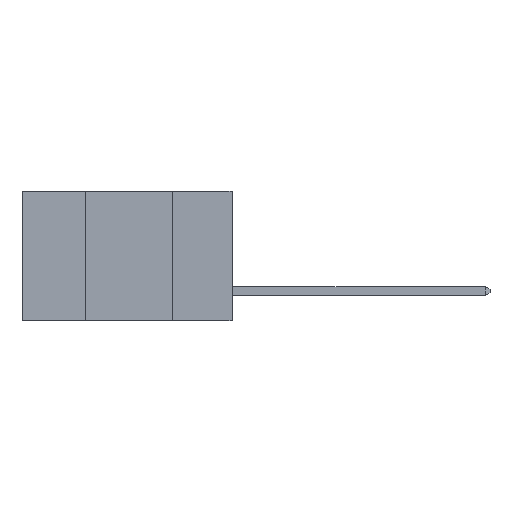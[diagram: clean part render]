
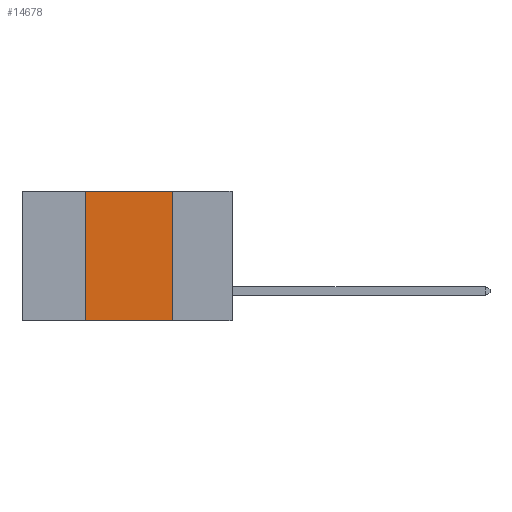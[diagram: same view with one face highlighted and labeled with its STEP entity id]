
A CAD part, left-side view. The second image highlights one B-rep face of the part: STEP entity #14678.
In plain terms, the highlighted planar face has unit normal (-1, 0, 0).
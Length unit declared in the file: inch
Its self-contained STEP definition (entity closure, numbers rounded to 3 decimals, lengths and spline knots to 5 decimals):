
#49 = DIRECTION ( 'NONE',  ( 0., -1., 0. ) ) ;
#316 = EDGE_CURVE ( 'NONE', #16548, #1294, #3854, .T. ) ;
#1294 = VERTEX_POINT ( 'NONE', #8686 ) ;
#1360 = ORIENTED_EDGE ( 'NONE', *, *, #15872, .F. ) ;
#1593 = LINE ( 'NONE', #1700, #14858 ) ;
#1700 = CARTESIAN_POINT ( 'NONE',  ( 0., 0.6, 0. ) ) ;
#1778 = VECTOR ( 'NONE', #7247, 39.37008 ) ;
#2514 = EDGE_LOOP ( 'NONE', ( #7907, #14664, #1360, #8323 ) ) ;
#3854 = LINE ( 'NONE', #7287, #13707 ) ;
#4302 = DIRECTION ( 'NONE',  ( 0., -1., 0. ) ) ;
#4315 = AXIS2_PLACEMENT_3D ( 'NONE', #5778, #14740, #7105 ) ;
#4480 = PLANE ( 'NONE',  #4315 ) ;
#5778 = CARTESIAN_POINT ( 'NONE',  ( 0., 0.6, 0. ) ) ;
#7105 = DIRECTION ( 'NONE',  ( 0., 0., -1. ) ) ;
#7247 = DIRECTION ( 'NONE',  ( 0., 0., 1. ) ) ;
#7287 = CARTESIAN_POINT ( 'NONE',  ( 0., 0.6, -0.37 ) ) ;
#7333 = CARTESIAN_POINT ( 'NONE',  ( 0., 0.42, 0. ) ) ;
#7784 = EDGE_CURVE ( 'NONE', #11010, #14756, #1593, .T. ) ;
#7906 = EDGE_CURVE ( 'NONE', #14756, #1294, #16605, .T. ) ;
#7907 = ORIENTED_EDGE ( 'NONE', *, *, #7906, .F. ) ;
#8169 = CARTESIAN_POINT ( 'NONE',  ( 0., 0.17, 0. ) ) ;
#8323 = ORIENTED_EDGE ( 'NONE', *, *, #316, .T. ) ;
#8686 = CARTESIAN_POINT ( 'NONE',  ( 0., 0.17, -0.37 ) ) ;
#11010 = VERTEX_POINT ( 'NONE', #7333 ) ;
#11124 = CARTESIAN_POINT ( 'NONE',  ( 0., 0.42, -0.37 ) ) ;
#11743 = FACE_OUTER_BOUND ( 'NONE', #2514, .T. ) ;
#12021 = DIRECTION ( 'NONE',  ( 0., 0., -1. ) ) ;
#12340 = CARTESIAN_POINT ( 'NONE',  ( 0., 0.42, 0. ) ) ;
#12374 = CARTESIAN_POINT ( 'NONE',  ( 0., 0.17, 0. ) ) ;
#12905 = VECTOR ( 'NONE', #12021, 39.37008 ) ;
#13707 = VECTOR ( 'NONE', #49, 39.37008 ) ;
#14664 = ORIENTED_EDGE ( 'NONE', *, *, #7784, .F. ) ;
#14678 = ADVANCED_FACE ( 'NONE', ( #11743 ), #4480, .F. ) ;
#14740 = DIRECTION ( 'NONE',  ( 1., 0., 0. ) ) ;
#14756 = VERTEX_POINT ( 'NONE', #12374 ) ;
#14858 = VECTOR ( 'NONE', #4302, 39.37008 ) ;
#15425 = LINE ( 'NONE', #12340, #1778 ) ;
#15872 = EDGE_CURVE ( 'NONE', #16548, #11010, #15425, .T. ) ;
#16548 = VERTEX_POINT ( 'NONE', #11124 ) ;
#16605 = LINE ( 'NONE', #8169, #12905 ) ;
